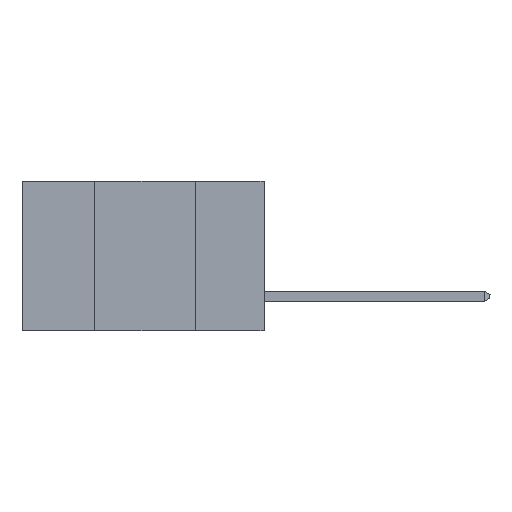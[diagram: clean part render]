
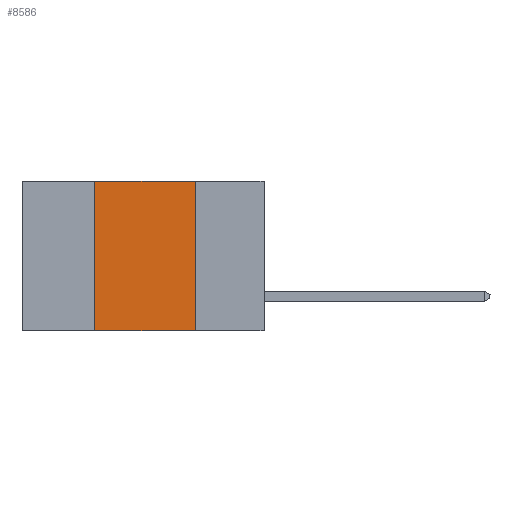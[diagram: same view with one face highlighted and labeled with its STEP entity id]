
A CAD part, left-side view. The second image highlights one B-rep face of the part: STEP entity #8586.
In plain terms, the highlighted planar face has unit normal (-1, 0, 0).
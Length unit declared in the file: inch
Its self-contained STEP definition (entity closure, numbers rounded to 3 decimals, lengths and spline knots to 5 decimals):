
#368 = PLANE ( 'NONE',  #9040 ) ;
#873 = ORIENTED_EDGE ( 'NONE', *, *, #10831, .F. ) ;
#1217 = VECTOR ( 'NONE', #9076, 39.37008 ) ;
#1478 = VERTEX_POINT ( 'NONE', #11398 ) ;
#1971 = VERTEX_POINT ( 'NONE', #5377 ) ;
#2298 = DIRECTION ( 'NONE',  ( 0., 0., -1. ) ) ;
#2559 = CARTESIAN_POINT ( 'NONE',  ( 0., 0.17, 0. ) ) ;
#2876 = EDGE_CURVE ( 'NONE', #1971, #1478, #6104, .T. ) ;
#2912 = VERTEX_POINT ( 'NONE', #10841 ) ;
#3033 = VERTEX_POINT ( 'NONE', #8669 ) ;
#3104 = EDGE_CURVE ( 'NONE', #2912, #3033, #5545, .T. ) ;
#3484 = ORIENTED_EDGE ( 'NONE', *, *, #7285, .T. ) ;
#3582 = EDGE_LOOP ( 'NONE', ( #4506, #873, #6401, #3484 ) ) ;
#3819 = FACE_OUTER_BOUND ( 'NONE', #3582, .T. ) ;
#4506 = ORIENTED_EDGE ( 'NONE', *, *, #3104, .F. ) ;
#4566 = CARTESIAN_POINT ( 'NONE',  ( 0., 0.6, -0.37 ) ) ;
#5265 = LINE ( 'NONE', #4566, #10884 ) ;
#5377 = CARTESIAN_POINT ( 'NONE',  ( 0., 0.42, -0.37 ) ) ;
#5461 = CARTESIAN_POINT ( 'NONE',  ( 0., 0.42, 0. ) ) ;
#5545 = LINE ( 'NONE', #2559, #11555 ) ;
#5986 = DIRECTION ( 'NONE',  ( 1., 0., 0. ) ) ;
#6104 = LINE ( 'NONE', #5461, #1217 ) ;
#6401 = ORIENTED_EDGE ( 'NONE', *, *, #2876, .F. ) ;
#7285 = EDGE_CURVE ( 'NONE', #1971, #3033, #5265, .T. ) ;
#7794 = DIRECTION ( 'NONE',  ( 0., -1., 0. ) ) ;
#8256 = LINE ( 'NONE', #10436, #9088 ) ;
#8586 = ADVANCED_FACE ( 'NONE', ( #3819 ), #368, .F. ) ;
#8616 = CARTESIAN_POINT ( 'NONE',  ( 0., 0.6, 0. ) ) ;
#8669 = CARTESIAN_POINT ( 'NONE',  ( 0., 0.17, -0.37 ) ) ;
#8902 = DIRECTION ( 'NONE',  ( 0., 0., -1. ) ) ;
#9040 = AXIS2_PLACEMENT_3D ( 'NONE', #8616, #5986, #2298 ) ;
#9076 = DIRECTION ( 'NONE',  ( 0., 0., 1. ) ) ;
#9088 = VECTOR ( 'NONE', #7794, 39.37008 ) ;
#9141 = DIRECTION ( 'NONE',  ( 0., -1., 0. ) ) ;
#10436 = CARTESIAN_POINT ( 'NONE',  ( 0., 0.6, 0. ) ) ;
#10831 = EDGE_CURVE ( 'NONE', #1478, #2912, #8256, .T. ) ;
#10841 = CARTESIAN_POINT ( 'NONE',  ( 0., 0.17, 0. ) ) ;
#10884 = VECTOR ( 'NONE', #9141, 39.37008 ) ;
#11398 = CARTESIAN_POINT ( 'NONE',  ( 0., 0.42, 0. ) ) ;
#11555 = VECTOR ( 'NONE', #8902, 39.37008 ) ;
